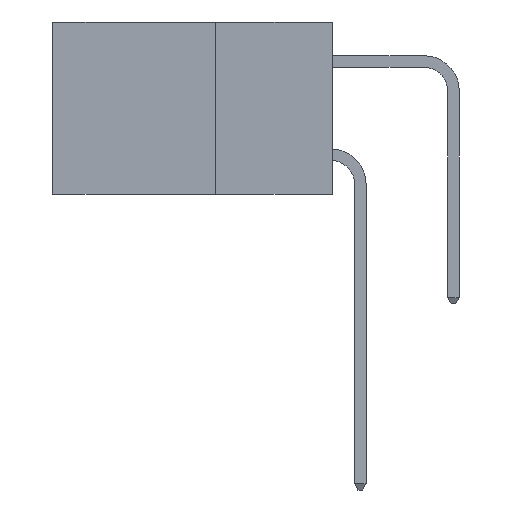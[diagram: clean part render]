
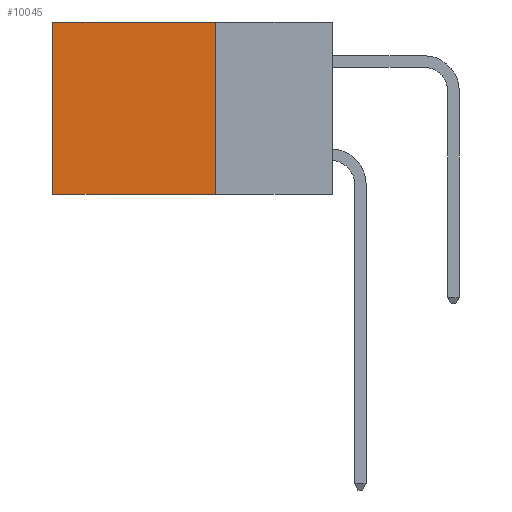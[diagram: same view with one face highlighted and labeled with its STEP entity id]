
A CAD part, left-side view. The second image highlights one B-rep face of the part: STEP entity #10045.
In plain terms, the highlighted planar face has unit normal (-1, 0, 0).
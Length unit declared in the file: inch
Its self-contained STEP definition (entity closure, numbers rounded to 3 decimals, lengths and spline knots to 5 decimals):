
#730 = LINE ( 'NONE', #9618, #5429 ) ;
#857 = DIRECTION ( 'NONE',  ( 0., 0., -1. ) ) ;
#1312 = DIRECTION ( 'NONE',  ( 0., 0., -1. ) ) ;
#2108 = DIRECTION ( 'NONE',  ( 0., 1., 0. ) ) ;
#2853 = VECTOR ( 'NONE', #857, 39.37008 ) ;
#3069 = EDGE_CURVE ( 'NONE', #5462, #8613, #10766, .T. ) ;
#3452 = VECTOR ( 'NONE', #10940, 39.37008 ) ;
#3865 = VERTEX_POINT ( 'NONE', #9807 ) ;
#4558 = ORIENTED_EDGE ( 'NONE', *, *, #6227, .F. ) ;
#4674 = ORIENTED_EDGE ( 'NONE', *, *, #10261, .T. ) ;
#4749 = LINE ( 'NONE', #7468, #2853 ) ;
#4960 = DIRECTION ( 'NONE',  ( 0., 0., -1. ) ) ;
#5429 = VECTOR ( 'NONE', #2108, 39.37008 ) ;
#5462 = VERTEX_POINT ( 'NONE', #7613 ) ;
#6140 = VECTOR ( 'NONE', #4960, 39.37008 ) ;
#6227 = EDGE_CURVE ( 'NONE', #3865, #8613, #730, .T. ) ;
#6983 = DIRECTION ( 'NONE',  ( 1., 0., 0. ) ) ;
#7468 = CARTESIAN_POINT ( 'NONE',  ( 0.2615, 0.25, -0.37 ) ) ;
#7613 = CARTESIAN_POINT ( 'NONE',  ( 0.2615, 0.6, 0. ) ) ;
#7760 = ORIENTED_EDGE ( 'NONE', *, *, #3069, .T. ) ;
#7902 = VERTEX_POINT ( 'NONE', #11710 ) ;
#8325 = ORIENTED_EDGE ( 'NONE', *, *, #10361, .F. ) ;
#8414 = EDGE_LOOP ( 'NONE', ( #7760, #4558, #8325, #4674 ) ) ;
#8613 = VERTEX_POINT ( 'NONE', #9927 ) ;
#8816 = PLANE ( 'NONE',  #11235 ) ;
#9618 = CARTESIAN_POINT ( 'NONE',  ( 0.2615, 0.25, -0.37 ) ) ;
#9807 = CARTESIAN_POINT ( 'NONE',  ( 0.2615, 0.25, -0.37 ) ) ;
#9927 = CARTESIAN_POINT ( 'NONE',  ( 0.2615, 0.6, -0.37 ) ) ;
#10045 = ADVANCED_FACE ( 'NONE', ( #11023 ), #8816, .F. ) ;
#10261 = EDGE_CURVE ( 'NONE', #7902, #5462, #10867, .T. ) ;
#10361 = EDGE_CURVE ( 'NONE', #7902, #3865, #4749, .T. ) ;
#10766 = LINE ( 'NONE', #11433, #6140 ) ;
#10867 = LINE ( 'NONE', #11847, #3452 ) ;
#10940 = DIRECTION ( 'NONE',  ( 0., 1., 0. ) ) ;
#11023 = FACE_OUTER_BOUND ( 'NONE', #8414, .T. ) ;
#11235 = AXIS2_PLACEMENT_3D ( 'NONE', #11530, #6983, #1312 ) ;
#11433 = CARTESIAN_POINT ( 'NONE',  ( 0.2615, 0.6, -0.37 ) ) ;
#11530 = CARTESIAN_POINT ( 'NONE',  ( 0.2615, 0.25, -0.37 ) ) ;
#11710 = CARTESIAN_POINT ( 'NONE',  ( 0.2615, 0.25, 0. ) ) ;
#11847 = CARTESIAN_POINT ( 'NONE',  ( 0.2615, 0.25, 0. ) ) ;
